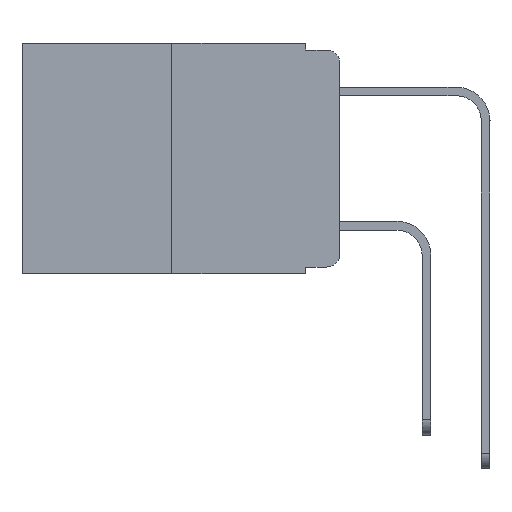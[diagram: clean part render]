
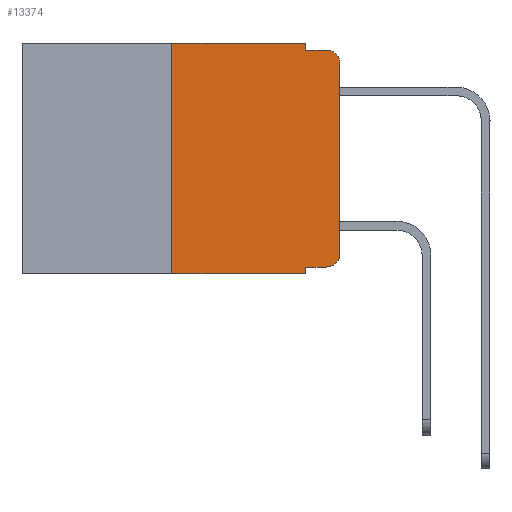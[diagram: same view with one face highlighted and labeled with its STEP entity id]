
A CAD part, left-side view. The second image highlights one B-rep face of the part: STEP entity #13374.
In plain terms, the highlighted planar face has unit normal (-1, 0, 0).
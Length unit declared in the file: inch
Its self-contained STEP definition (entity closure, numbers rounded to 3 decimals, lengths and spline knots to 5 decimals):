
#86 = LINE ( 'NONE', #237, #5094 ) ;
#92 = LINE ( 'NONE', #4249, #10598 ) ;
#237 = CARTESIAN_POINT ( 'NONE',  ( 0., 0.25, 0. ) ) ;
#284 = LINE ( 'NONE', #18656, #21201 ) ;
#792 = EDGE_CURVE ( 'NONE', #3414, #15990, #20821, .T. ) ;
#885 = ORIENTED_EDGE ( 'NONE', *, *, #7347, .T. ) ;
#1615 = ORIENTED_EDGE ( 'NONE', *, *, #12877, .T. ) ;
#2832 = VERTEX_POINT ( 'NONE', #9578 ) ;
#3267 = ORIENTED_EDGE ( 'NONE', *, *, #6987, .F. ) ;
#3270 = DIRECTION ( 'NONE',  ( 0., -1., 0. ) ) ;
#3414 = VERTEX_POINT ( 'NONE', #12258 ) ;
#3574 = DIRECTION ( 'NONE',  ( 1., 0., 0. ) ) ;
#3927 = CARTESIAN_POINT ( 'NONE',  ( 0., 0.02, -0.313 ) ) ;
#3943 = EDGE_CURVE ( 'NONE', #4314, #9465, #21014, .T. ) ;
#4013 = VECTOR ( 'NONE', #8816, 39.37008 ) ;
#4055 = CARTESIAN_POINT ( 'NONE',  ( 0., 0.25, -0.343 ) ) ;
#4249 = CARTESIAN_POINT ( 'NONE',  ( 0., 0.051, 0. ) ) ;
#4314 = VERTEX_POINT ( 'NONE', #20329 ) ;
#4930 = CARTESIAN_POINT ( 'NONE',  ( 0., 0.051, -0.333 ) ) ;
#5094 = VECTOR ( 'NONE', #16989, 39.37008 ) ;
#5141 = ORIENTED_EDGE ( 'NONE', *, *, #792, .F. ) ;
#5595 = CARTESIAN_POINT ( 'NONE',  ( 0., 0.051, -0.343 ) ) ;
#5694 = DIRECTION ( 'NONE',  ( 0., 0., -1. ) ) ;
#6086 = DIRECTION ( 'NONE',  ( 0., 0., -1. ) ) ;
#6963 = VERTEX_POINT ( 'NONE', #5595 ) ;
#6987 = EDGE_CURVE ( 'NONE', #2832, #3414, #21758, .T. ) ;
#7347 = EDGE_CURVE ( 'NONE', #21458, #15990, #17560, .T. ) ;
#7685 = CARTESIAN_POINT ( 'NONE',  ( 0., 0., -0.313 ) ) ;
#7976 = DIRECTION ( 'NONE',  ( 0., -1., 0. ) ) ;
#8454 = DIRECTION ( 'NONE',  ( 0., 0., -1. ) ) ;
#8675 = EDGE_CURVE ( 'NONE', #22967, #6963, #13861, .T. ) ;
#8816 = DIRECTION ( 'NONE',  ( 0., -1., 0. ) ) ;
#9068 = AXIS2_PLACEMENT_3D ( 'NONE', #13937, #3574, #18187 ) ;
#9465 = VERTEX_POINT ( 'NONE', #12495 ) ;
#9578 = CARTESIAN_POINT ( 'NONE',  ( 0., 0.051, 0. ) ) ;
#9936 = VECTOR ( 'NONE', #3270, 39.37008 ) ;
#10559 = CARTESIAN_POINT ( 'NONE',  ( 0., 0.25, 0. ) ) ;
#10598 = VECTOR ( 'NONE', #8454, 39.37008 ) ;
#11028 = AXIS2_PLACEMENT_3D ( 'NONE', #19657, #15353, #12956 ) ;
#11197 = CIRCLE ( 'NONE', #12953, 0.02 ) ;
#11860 = PLANE ( 'NONE',  #9068 ) ;
#12258 = CARTESIAN_POINT ( 'NONE',  ( 0., 0.051, -0.01 ) ) ;
#12495 = CARTESIAN_POINT ( 'NONE',  ( 0., 0.02, -0.333 ) ) ;
#12877 = EDGE_CURVE ( 'NONE', #17565, #21458, #284, .T. ) ;
#12953 = AXIS2_PLACEMENT_3D ( 'NONE', #3927, #18547, #6086 ) ;
#12956 = DIRECTION ( 'NONE',  ( 0., 0., -1. ) ) ;
#13374 = ADVANCED_FACE ( 'NONE', ( #20546 ), #11860, .F. ) ;
#13796 = CARTESIAN_POINT ( 'NONE',  ( 0., 0.051, -0.01 ) ) ;
#13861 = LINE ( 'NONE', #18326, #22942 ) ;
#13937 = CARTESIAN_POINT ( 'NONE',  ( 0., 0.473, 0. ) ) ;
#14997 = CARTESIAN_POINT ( 'NONE',  ( 0., 0.473, 0. ) ) ;
#15291 = VECTOR ( 'NONE', #7976, 39.37008 ) ;
#15323 = EDGE_LOOP ( 'NONE', ( #1615, #885, #5141, #3267, #21196, #22334, #15372, #17412, #17577, #19101 ) ) ;
#15353 = DIRECTION ( 'NONE',  ( -1., 0., 0. ) ) ;
#15372 = ORIENTED_EDGE ( 'NONE', *, *, #8675, .T. ) ;
#15990 = VERTEX_POINT ( 'NONE', #24825 ) ;
#16026 = EDGE_CURVE ( 'NONE', #4314, #6963, #92, .T. ) ;
#16989 = DIRECTION ( 'NONE',  ( 0., 0., 1. ) ) ;
#17045 = EDGE_CURVE ( 'NONE', #9465, #17565, #11197, .T. ) ;
#17412 = ORIENTED_EDGE ( 'NONE', *, *, #16026, .F. ) ;
#17560 = CIRCLE ( 'NONE', #11028, 0.02 ) ;
#17565 = VERTEX_POINT ( 'NONE', #7685 ) ;
#17577 = ORIENTED_EDGE ( 'NONE', *, *, #3943, .T. ) ;
#17854 = CARTESIAN_POINT ( 'NONE',  ( 0., 0.051, 0. ) ) ;
#18187 = DIRECTION ( 'NONE',  ( 0., 0., -1. ) ) ;
#18326 = CARTESIAN_POINT ( 'NONE',  ( 0., 0.473, -0.343 ) ) ;
#18547 = DIRECTION ( 'NONE',  ( -1., 0., 0. ) ) ;
#18656 = CARTESIAN_POINT ( 'NONE',  ( 0., 0., 0. ) ) ;
#19101 = ORIENTED_EDGE ( 'NONE', *, *, #17045, .T. ) ;
#19426 = CARTESIAN_POINT ( 'NONE',  ( 0., 0., -0.03 ) ) ;
#19657 = CARTESIAN_POINT ( 'NONE',  ( 0., 0.02, -0.03 ) ) ;
#20068 = EDGE_CURVE ( 'NONE', #22967, #26701, #86, .T. ) ;
#20329 = CARTESIAN_POINT ( 'NONE',  ( 0., 0.051, -0.333 ) ) ;
#20546 = FACE_OUTER_BOUND ( 'NONE', #15323, .T. ) ;
#20656 = LINE ( 'NONE', #14997, #4013 ) ;
#20821 = LINE ( 'NONE', #13796, #15291 ) ;
#21014 = LINE ( 'NONE', #4930, #9936 ) ;
#21196 = ORIENTED_EDGE ( 'NONE', *, *, #21909, .F. ) ;
#21201 = VECTOR ( 'NONE', #24713, 39.37008 ) ;
#21458 = VERTEX_POINT ( 'NONE', #19426 ) ;
#21758 = LINE ( 'NONE', #17854, #26513 ) ;
#21909 = EDGE_CURVE ( 'NONE', #26701, #2832, #20656, .T. ) ;
#22334 = ORIENTED_EDGE ( 'NONE', *, *, #20068, .F. ) ;
#22942 = VECTOR ( 'NONE', #24488, 39.37008 ) ;
#22967 = VERTEX_POINT ( 'NONE', #4055 ) ;
#24488 = DIRECTION ( 'NONE',  ( 0., -1., 0. ) ) ;
#24713 = DIRECTION ( 'NONE',  ( 0., 0., 1. ) ) ;
#24825 = CARTESIAN_POINT ( 'NONE',  ( 0., 0.02, -0.01 ) ) ;
#26513 = VECTOR ( 'NONE', #5694, 39.37008 ) ;
#26701 = VERTEX_POINT ( 'NONE', #10559 ) ;
